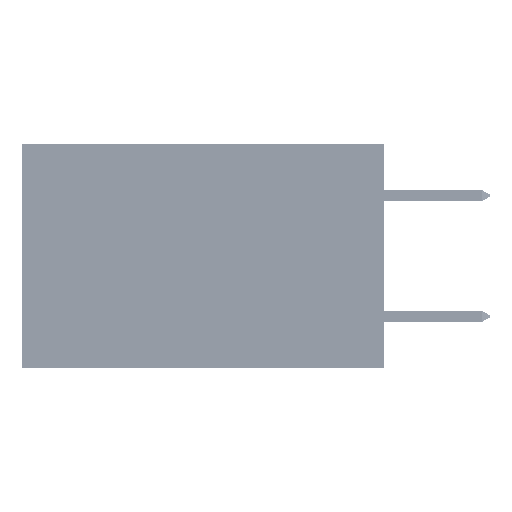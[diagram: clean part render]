
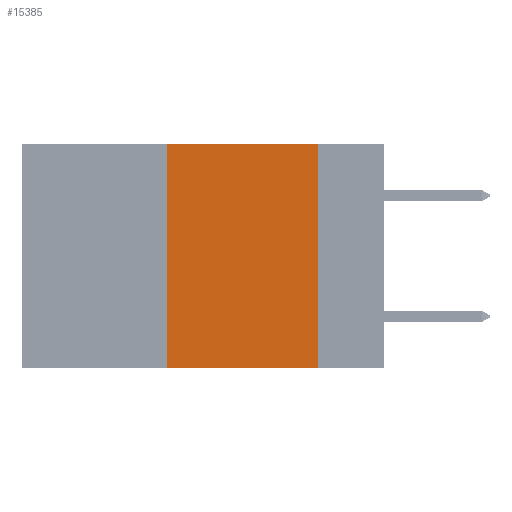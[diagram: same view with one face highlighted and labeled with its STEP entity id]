
A CAD part, left-side view. The second image highlights one B-rep face of the part: STEP entity #15385.
In plain terms, the highlighted planar face has unit normal (-1, 0, 0).
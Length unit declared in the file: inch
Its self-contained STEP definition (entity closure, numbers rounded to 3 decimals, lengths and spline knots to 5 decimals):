
#117 = DIRECTION ( 'NONE',  ( 0., -1., 0. ) ) ;
#1304 = VERTEX_POINT ( 'NONE', #19949 ) ;
#1637 = VECTOR ( 'NONE', #117, 39.37008 ) ;
#4799 = CARTESIAN_POINT ( 'NONE',  ( 0., 0.36, 0. ) ) ;
#6823 = VERTEX_POINT ( 'NONE', #13785 ) ;
#7294 = PLANE ( 'NONE',  #47409 ) ;
#9481 = CARTESIAN_POINT ( 'NONE',  ( 0., 0.11, 0. ) ) ;
#9770 = VECTOR ( 'NONE', #32968, 39.37008 ) ;
#10847 = EDGE_CURVE ( 'NONE', #1304, #6823, #27806, .T. ) ;
#11387 = CARTESIAN_POINT ( 'NONE',  ( 0., 0.6, 0. ) ) ;
#11663 = LINE ( 'NONE', #20306, #1637 ) ;
#12104 = VECTOR ( 'NONE', #35099, 39.37008 ) ;
#13784 = EDGE_LOOP ( 'NONE', ( #26839, #38727, #44188, #48357 ) ) ;
#13785 = CARTESIAN_POINT ( 'NONE',  ( 0., 0.36, 0. ) ) ;
#14635 = CARTESIAN_POINT ( 'NONE',  ( 0., 0.11, -0.37 ) ) ;
#15385 = ADVANCED_FACE ( 'NONE', ( #34382 ), #7294, .F. ) ;
#16405 = LINE ( 'NONE', #9481, #9770 ) ;
#19521 = LINE ( 'NONE', #27953, #12104 ) ;
#19949 = CARTESIAN_POINT ( 'NONE',  ( 0., 0.36, -0.37 ) ) ;
#20306 = CARTESIAN_POINT ( 'NONE',  ( 0., 0.6, 0. ) ) ;
#26839 = ORIENTED_EDGE ( 'NONE', *, *, #36463, .F. ) ;
#27806 = LINE ( 'NONE', #4799, #37290 ) ;
#27953 = CARTESIAN_POINT ( 'NONE',  ( 0., 0.6, -0.37 ) ) ;
#30073 = VERTEX_POINT ( 'NONE', #14635 ) ;
#32968 = DIRECTION ( 'NONE',  ( 0., 0., -1. ) ) ;
#33793 = CARTESIAN_POINT ( 'NONE',  ( 0., 0.11, 0. ) ) ;
#34382 = FACE_OUTER_BOUND ( 'NONE', #13784, .T. ) ;
#35099 = DIRECTION ( 'NONE',  ( 0., -1., 0. ) ) ;
#36209 = DIRECTION ( 'NONE',  ( 0., 0., 1. ) ) ;
#36463 = EDGE_CURVE ( 'NONE', #40971, #30073, #16405, .T. ) ;
#37290 = VECTOR ( 'NONE', #36209, 39.37008 ) ;
#38723 = DIRECTION ( 'NONE',  ( 0., 0., -1. ) ) ;
#38727 = ORIENTED_EDGE ( 'NONE', *, *, #48341, .F. ) ;
#40971 = VERTEX_POINT ( 'NONE', #33793 ) ;
#43570 = EDGE_CURVE ( 'NONE', #1304, #30073, #19521, .T. ) ;
#44188 = ORIENTED_EDGE ( 'NONE', *, *, #10847, .F. ) ;
#47409 = AXIS2_PLACEMENT_3D ( 'NONE', #11387, #50530, #38723 ) ;
#48341 = EDGE_CURVE ( 'NONE', #6823, #40971, #11663, .T. ) ;
#48357 = ORIENTED_EDGE ( 'NONE', *, *, #43570, .T. ) ;
#50530 = DIRECTION ( 'NONE',  ( 1., 0., 0. ) ) ;
